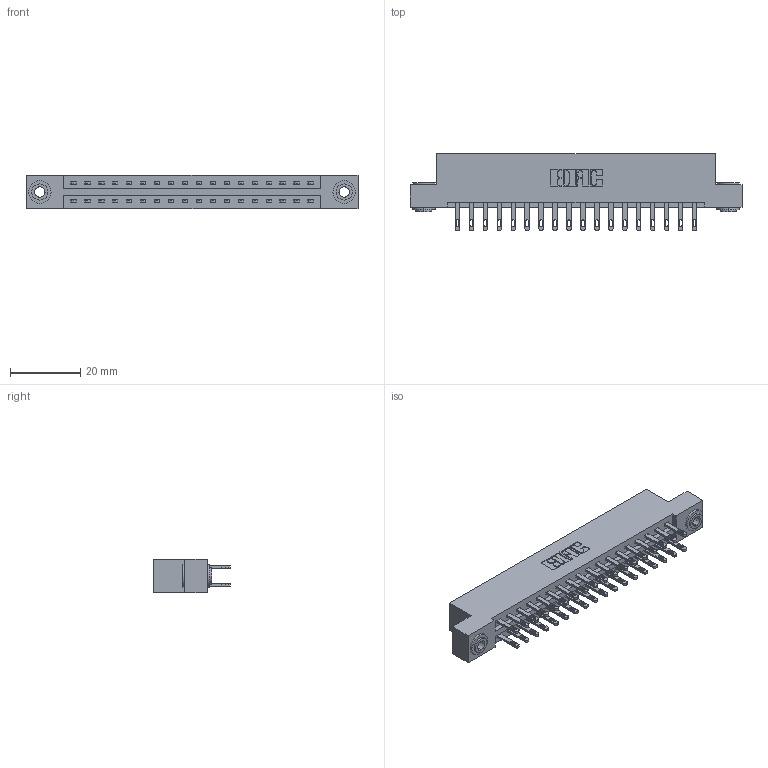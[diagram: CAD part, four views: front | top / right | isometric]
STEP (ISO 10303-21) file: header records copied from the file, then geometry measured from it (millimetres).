
FILE_DESCRIPTION (( 'STEP AP203' ), '1' );
FILE_NAME ('337-036-500-203.STEP', '2019-10-08T20:32:55', ( '' ), ( '' ), 'SwSTEP 2.0', 'SolidWorks 2016', '' );
FILE_SCHEMA (( 'CONFIG_CONTROL_DESIGN' ));
Length unit declared in the file: inch
Products named in the file (4): 345-250-002_345-250-002-102; 337-036-500-203; 345-292-001_345-293-100; 337 Part_Flush Mounting Lugs - 0.156 Dia-TH
Assembly tree (39 placements, depth 2):
  337-036-500-203
    337 Part_Flush Mounting Lugs - 0.156 Dia-TH
    345-292-001_345-293-100  x36
    345-250-002_345-250-002-102  x2
Bounding box: 94.34 x 21.85 x 9.4 mm (x, y, z)
Volume: 9751.8 mm3; surface area: 11415.1 mm2
Topology: 39 solids, 39 shells, 1952 faces, 5895 edges, 3926 vertices
Faces by surface type: plane 1232, cylinder 712, cone 8
Entity records: 17640 total; most frequent: CARTESIAN_POINT 2965, ORIENTED_EDGE 2894, DIRECTION 2601, EDGE_CURVE 1447, VECTOR 1291, LINE 1291, VERTEX_POINT 962, AXIS2_PLACEMENT_3D 655
